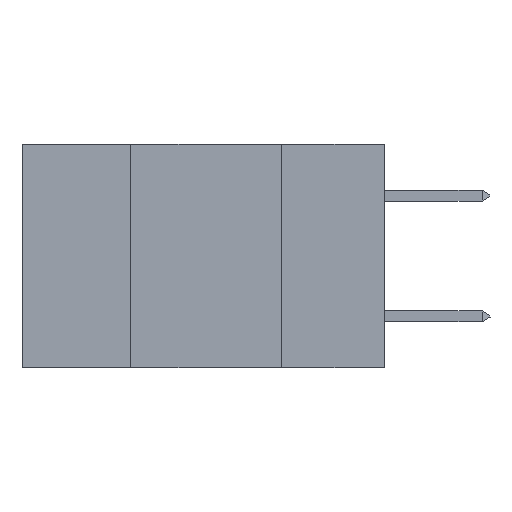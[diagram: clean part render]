
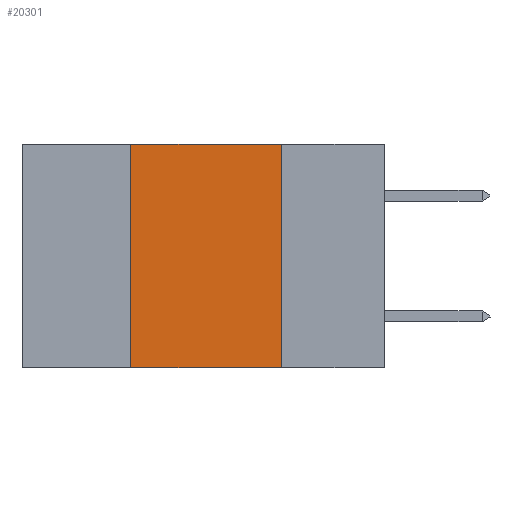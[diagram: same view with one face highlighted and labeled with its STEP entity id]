
A CAD part, left-side view. The second image highlights one B-rep face of the part: STEP entity #20301.
In plain terms, the highlighted planar face has unit normal (-1, 0, 0).
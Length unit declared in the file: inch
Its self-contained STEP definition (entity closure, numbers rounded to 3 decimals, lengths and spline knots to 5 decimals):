
#893 = DIRECTION ( 'NONE',  ( 0., -1., 0. ) ) ;
#1341 = CARTESIAN_POINT ( 'NONE',  ( 0., 0.6, 0. ) ) ;
#2196 = VECTOR ( 'NONE', #39880, 39.37008 ) ;
#2781 = EDGE_CURVE ( 'NONE', #38841, #31279, #14055, .T. ) ;
#4568 = VECTOR ( 'NONE', #893, 39.37008 ) ;
#6167 = EDGE_CURVE ( 'NONE', #15271, #31971, #22251, .T. ) ;
#7257 = CARTESIAN_POINT ( 'NONE',  ( 0., 0.17, 0. ) ) ;
#10562 = CARTESIAN_POINT ( 'NONE',  ( 0., 0.42, 0. ) ) ;
#10608 = CARTESIAN_POINT ( 'NONE',  ( 0., 0.6, -0.37 ) ) ;
#13922 = DIRECTION ( 'NONE',  ( 0., 0., -1. ) ) ;
#14055 = LINE ( 'NONE', #10608, #28627 ) ;
#15271 = VERTEX_POINT ( 'NONE', #10562 ) ;
#16263 = ORIENTED_EDGE ( 'NONE', *, *, #2781, .T. ) ;
#19189 = ORIENTED_EDGE ( 'NONE', *, *, #43010, .F. ) ;
#19252 = VECTOR ( 'NONE', #13922, 39.37008 ) ;
#19368 = AXIS2_PLACEMENT_3D ( 'NONE', #29719, #33836, #40286 ) ;
#20089 = PLANE ( 'NONE',  #19368 ) ;
#20301 = ADVANCED_FACE ( 'NONE', ( #26518 ), #20089, .F. ) ;
#22251 = LINE ( 'NONE', #1341, #4568 ) ;
#25895 = LINE ( 'NONE', #32291, #2196 ) ;
#26518 = FACE_OUTER_BOUND ( 'NONE', #32983, .T. ) ;
#28389 = CARTESIAN_POINT ( 'NONE',  ( 0., 0.17, 0. ) ) ;
#28627 = VECTOR ( 'NONE', #31698, 39.37008 ) ;
#29719 = CARTESIAN_POINT ( 'NONE',  ( 0., 0.6, 0. ) ) ;
#31279 = VERTEX_POINT ( 'NONE', #39949 ) ;
#31698 = DIRECTION ( 'NONE',  ( 0., -1., 0. ) ) ;
#31971 = VERTEX_POINT ( 'NONE', #28389 ) ;
#32291 = CARTESIAN_POINT ( 'NONE',  ( 0., 0.42, 0. ) ) ;
#32782 = LINE ( 'NONE', #7257, #19252 ) ;
#32983 = EDGE_LOOP ( 'NONE', ( #19189, #33145, #42889, #16263 ) ) ;
#33145 = ORIENTED_EDGE ( 'NONE', *, *, #6167, .F. ) ;
#33836 = DIRECTION ( 'NONE',  ( 1., 0., 0. ) ) ;
#35290 = CARTESIAN_POINT ( 'NONE',  ( 0., 0.42, -0.37 ) ) ;
#38841 = VERTEX_POINT ( 'NONE', #35290 ) ;
#39880 = DIRECTION ( 'NONE',  ( 0., 0., 1. ) ) ;
#39949 = CARTESIAN_POINT ( 'NONE',  ( 0., 0.17, -0.37 ) ) ;
#40286 = DIRECTION ( 'NONE',  ( 0., 0., -1. ) ) ;
#40306 = EDGE_CURVE ( 'NONE', #38841, #15271, #25895, .T. ) ;
#42889 = ORIENTED_EDGE ( 'NONE', *, *, #40306, .F. ) ;
#43010 = EDGE_CURVE ( 'NONE', #31971, #31279, #32782, .T. ) ;
